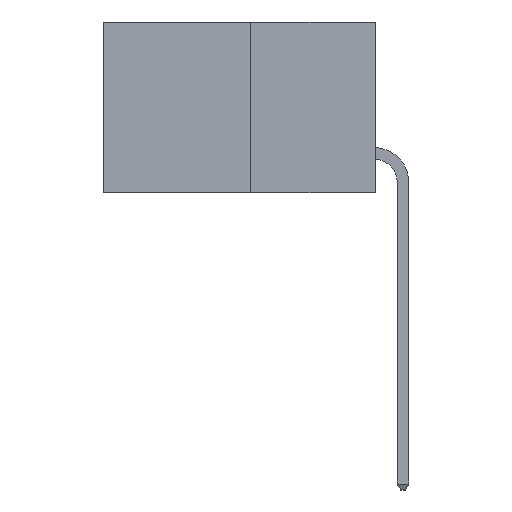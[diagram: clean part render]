
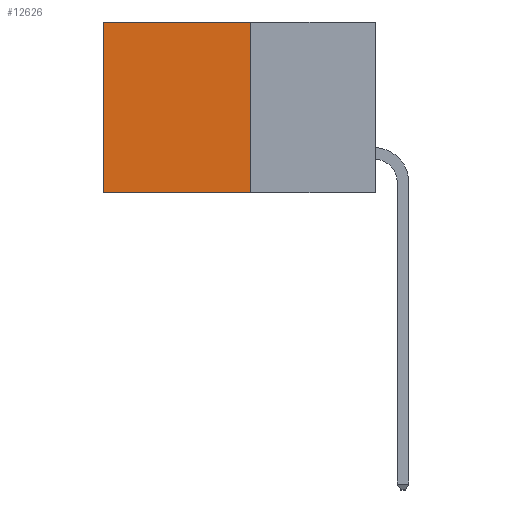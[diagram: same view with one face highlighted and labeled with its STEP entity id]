
A CAD part, left-side view. The second image highlights one B-rep face of the part: STEP entity #12626.
In plain terms, the highlighted planar face has unit normal (-1, 0, 0).
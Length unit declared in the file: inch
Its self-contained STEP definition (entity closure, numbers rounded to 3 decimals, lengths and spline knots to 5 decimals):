
#368 = VERTEX_POINT ( 'NONE', #6761 ) ;
#592 = EDGE_CURVE ( 'NONE', #3291, #368, #7833, .T. ) ;
#809 = CARTESIAN_POINT ( 'NONE',  ( 0.277, 0.27, 0. ) ) ;
#864 = DIRECTION ( 'NONE',  ( 0., 1., 0. ) ) ;
#1295 = VERTEX_POINT ( 'NONE', #11322 ) ;
#1722 = DIRECTION ( 'NONE',  ( 0., 0., -1. ) ) ;
#1799 = ORIENTED_EDGE ( 'NONE', *, *, #592, .F. ) ;
#2147 = VECTOR ( 'NONE', #1722, 39.37008 ) ;
#2160 = FACE_OUTER_BOUND ( 'NONE', #8410, .T. ) ;
#2325 = CARTESIAN_POINT ( 'NONE',  ( 0.277, 0.59, -0.37 ) ) ;
#3291 = VERTEX_POINT ( 'NONE', #7397 ) ;
#4076 = CARTESIAN_POINT ( 'NONE',  ( 0.277, 0.27, -0.37 ) ) ;
#4195 = DIRECTION ( 'NONE',  ( 0., 1., 0. ) ) ;
#4336 = LINE ( 'NONE', #809, #9285 ) ;
#4401 = EDGE_CURVE ( 'NONE', #12957, #1295, #7061, .T. ) ;
#5418 = DIRECTION ( 'NONE',  ( 1., 0., 0. ) ) ;
#6362 = PLANE ( 'NONE',  #12127 ) ;
#6678 = ORIENTED_EDGE ( 'NONE', *, *, #7955, .F. ) ;
#6761 = CARTESIAN_POINT ( 'NONE',  ( 0.277, 0.27, -0.37 ) ) ;
#6778 = VECTOR ( 'NONE', #10455, 39.37008 ) ;
#6815 = CARTESIAN_POINT ( 'NONE',  ( 0.277, 0.59, 0. ) ) ;
#7061 = LINE ( 'NONE', #2325, #6778 ) ;
#7113 = VECTOR ( 'NONE', #4195, 39.37008 ) ;
#7397 = CARTESIAN_POINT ( 'NONE',  ( 0.277, 0.27, 0. ) ) ;
#7779 = ORIENTED_EDGE ( 'NONE', *, *, #4401, .T. ) ;
#7793 = EDGE_CURVE ( 'NONE', #3291, #12957, #4336, .T. ) ;
#7833 = LINE ( 'NONE', #11684, #2147 ) ;
#7955 = EDGE_CURVE ( 'NONE', #368, #1295, #9766, .T. ) ;
#8410 = EDGE_LOOP ( 'NONE', ( #7779, #6678, #1799, #8858 ) ) ;
#8858 = ORIENTED_EDGE ( 'NONE', *, *, #7793, .T. ) ;
#9285 = VECTOR ( 'NONE', #864, 39.37008 ) ;
#9766 = LINE ( 'NONE', #4076, #7113 ) ;
#10455 = DIRECTION ( 'NONE',  ( 0., 0., -1. ) ) ;
#11322 = CARTESIAN_POINT ( 'NONE',  ( 0.277, 0.59, -0.37 ) ) ;
#11324 = CARTESIAN_POINT ( 'NONE',  ( 0.277, 0.27, -0.37 ) ) ;
#11684 = CARTESIAN_POINT ( 'NONE',  ( 0.277, 0.27, -0.37 ) ) ;
#12127 = AXIS2_PLACEMENT_3D ( 'NONE', #11324, #5418, #12315 ) ;
#12315 = DIRECTION ( 'NONE',  ( 0., 0., -1. ) ) ;
#12626 = ADVANCED_FACE ( 'NONE', ( #2160 ), #6362, .F. ) ;
#12957 = VERTEX_POINT ( 'NONE', #6815 ) ;
